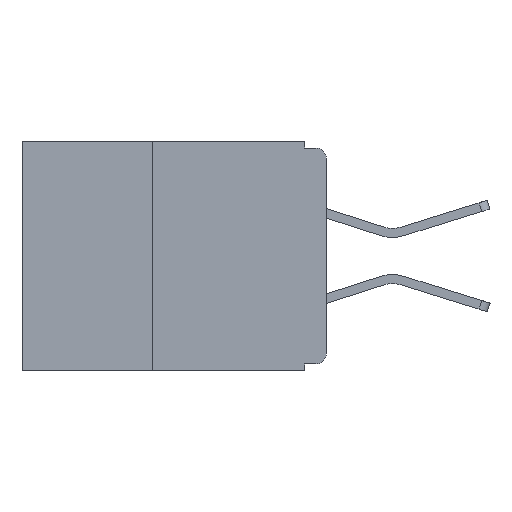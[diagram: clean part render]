
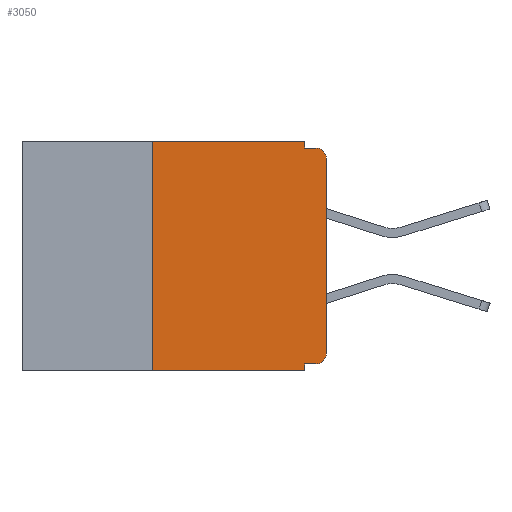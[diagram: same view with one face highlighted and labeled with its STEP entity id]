
A CAD part, left-side view. The second image highlights one B-rep face of the part: STEP entity #3050.
In plain terms, the highlighted planar face has unit normal (-1, 0, 0).
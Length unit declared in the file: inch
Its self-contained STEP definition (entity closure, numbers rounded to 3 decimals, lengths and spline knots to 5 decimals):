
#197 = ORIENTED_EDGE ( 'NONE', *, *, #4888, .F. ) ;
#279 = CARTESIAN_POINT ( 'NONE',  ( 0., 0., -0.01 ) ) ;
#419 = CARTESIAN_POINT ( 'NONE',  ( 0., 0.437, -0.33 ) ) ;
#946 = ORIENTED_EDGE ( 'NONE', *, *, #11681, .T. ) ;
#1035 = VERTEX_POINT ( 'NONE', #1545 ) ;
#1174 = VERTEX_POINT ( 'NONE', #5478 ) ;
#1200 = LINE ( 'NONE', #7722, #11026 ) ;
#1392 = EDGE_CURVE ( 'NONE', #10368, #1035, #6791, .T. ) ;
#1545 = CARTESIAN_POINT ( 'NONE',  ( 0., 0.015, -0.01 ) ) ;
#1683 = CARTESIAN_POINT ( 'NONE',  ( 0., 0., 0. ) ) ;
#1817 = ORIENTED_EDGE ( 'NONE', *, *, #6725, .F. ) ;
#1857 = CARTESIAN_POINT ( 'NONE',  ( 0., 0.437, 0. ) ) ;
#1884 = ORIENTED_EDGE ( 'NONE', *, *, #3184, .F. ) ;
#2213 = DIRECTION ( 'NONE',  ( 0., 0., -1. ) ) ;
#2411 = AXIS2_PLACEMENT_3D ( 'NONE', #9048, #4273, #4188 ) ;
#2417 = CARTESIAN_POINT ( 'NONE',  ( 0., 0., -0.305 ) ) ;
#2438 = CARTESIAN_POINT ( 'NONE',  ( 0., 0.015, -0.32 ) ) ;
#2534 = CARTESIAN_POINT ( 'NONE',  ( 0., 0.031, 0. ) ) ;
#2611 = DIRECTION ( 'NONE',  ( 0., 0., 1. ) ) ;
#2710 = DIRECTION ( 'NONE',  ( 0., 0., -1. ) ) ;
#3050 = ADVANCED_FACE ( 'NONE', ( #4668 ), #9510, .F. ) ;
#3118 = LINE ( 'NONE', #7141, #7321 ) ;
#3184 = EDGE_CURVE ( 'NONE', #4792, #7327, #10621, .T. ) ;
#3186 = AXIS2_PLACEMENT_3D ( 'NONE', #1857, #9550, #2710 ) ;
#3402 = AXIS2_PLACEMENT_3D ( 'NONE', #7175, #7923, #2213 ) ;
#3462 = ORIENTED_EDGE ( 'NONE', *, *, #9249, .T. ) ;
#3850 = CARTESIAN_POINT ( 'NONE',  ( 0., 0., -0.025 ) ) ;
#3907 = LINE ( 'NONE', #419, #4951 ) ;
#4050 = DIRECTION ( 'NONE',  ( 0., 1., 0. ) ) ;
#4117 = CARTESIAN_POINT ( 'NONE',  ( 0., 0.25, -0.33 ) ) ;
#4188 = DIRECTION ( 'NONE',  ( 0., 0., -1. ) ) ;
#4189 = DIRECTION ( 'NONE',  ( 0., -1., 0. ) ) ;
#4273 = DIRECTION ( 'NONE',  ( -1., 0., 0. ) ) ;
#4319 = DIRECTION ( 'NONE',  ( 0., 0., 1. ) ) ;
#4668 = FACE_OUTER_BOUND ( 'NONE', #10624, .T. ) ;
#4792 = VERTEX_POINT ( 'NONE', #7662 ) ;
#4888 = EDGE_CURVE ( 'NONE', #9612, #1174, #6594, .T. ) ;
#4899 = DIRECTION ( 'NONE',  ( 0., 0., -1. ) ) ;
#4951 = VECTOR ( 'NONE', #7119, 39.37008 ) ;
#5375 = VECTOR ( 'NONE', #2611, 39.37008 ) ;
#5478 = CARTESIAN_POINT ( 'NONE',  ( 0., 0.031, -0.32 ) ) ;
#5643 = EDGE_CURVE ( 'NONE', #7419, #12080, #8805, .T. ) ;
#5899 = EDGE_CURVE ( 'NONE', #11147, #4792, #3118, .T. ) ;
#6088 = CARTESIAN_POINT ( 'NONE',  ( 0., 0.031, -0.33 ) ) ;
#6113 = LINE ( 'NONE', #6088, #10429 ) ;
#6269 = CARTESIAN_POINT ( 'NONE',  ( 0., 0.031, -0.33 ) ) ;
#6420 = CIRCLE ( 'NONE', #2411, 0.015 ) ;
#6594 = LINE ( 'NONE', #10680, #10911 ) ;
#6725 = EDGE_CURVE ( 'NONE', #7327, #10368, #1200, .T. ) ;
#6791 = LINE ( 'NONE', #279, #8722 ) ;
#6833 = VERTEX_POINT ( 'NONE', #6269 ) ;
#6882 = DIRECTION ( 'NONE',  ( 0., -1., 0. ) ) ;
#6941 = CIRCLE ( 'NONE', #3402, 0.015 ) ;
#7119 = DIRECTION ( 'NONE',  ( 0., -1., 0. ) ) ;
#7141 = CARTESIAN_POINT ( 'NONE',  ( 0., 0.25, -0.33 ) ) ;
#7151 = ORIENTED_EDGE ( 'NONE', *, *, #1392, .F. ) ;
#7175 = CARTESIAN_POINT ( 'NONE',  ( 0., 0.015, -0.025 ) ) ;
#7182 = DIRECTION ( 'NONE',  ( 0., 0., -1. ) ) ;
#7321 = VECTOR ( 'NONE', #4319, 39.37008 ) ;
#7327 = VERTEX_POINT ( 'NONE', #2534 ) ;
#7419 = VERTEX_POINT ( 'NONE', #2417 ) ;
#7545 = ORIENTED_EDGE ( 'NONE', *, *, #5899, .F. ) ;
#7566 = ORIENTED_EDGE ( 'NONE', *, *, #11706, .F. ) ;
#7662 = CARTESIAN_POINT ( 'NONE',  ( 0., 0.25, 0. ) ) ;
#7676 = ORIENTED_EDGE ( 'NONE', *, *, #5643, .T. ) ;
#7722 = CARTESIAN_POINT ( 'NONE',  ( 0., 0.031, 0. ) ) ;
#7873 = CARTESIAN_POINT ( 'NONE',  ( 0., 0.031, -0.01 ) ) ;
#7923 = DIRECTION ( 'NONE',  ( -1., 0., 0. ) ) ;
#8722 = VECTOR ( 'NONE', #4189, 39.37008 ) ;
#8805 = LINE ( 'NONE', #1683, #5375 ) ;
#9048 = CARTESIAN_POINT ( 'NONE',  ( 0., 0.015, -0.305 ) ) ;
#9249 = EDGE_CURVE ( 'NONE', #12080, #1035, #6941, .T. ) ;
#9510 = PLANE ( 'NONE',  #3186 ) ;
#9550 = DIRECTION ( 'NONE',  ( 1., 0., 0. ) ) ;
#9612 = VERTEX_POINT ( 'NONE', #2438 ) ;
#10368 = VERTEX_POINT ( 'NONE', #7873 ) ;
#10429 = VECTOR ( 'NONE', #7182, 39.37008 ) ;
#10468 = EDGE_CURVE ( 'NONE', #11147, #6833, #3907, .T. ) ;
#10546 = ORIENTED_EDGE ( 'NONE', *, *, #10468, .T. ) ;
#10621 = LINE ( 'NONE', #11627, #11976 ) ;
#10624 = EDGE_LOOP ( 'NONE', ( #7676, #3462, #7151, #1817, #1884, #7545, #10546, #7566, #197, #946 ) ) ;
#10680 = CARTESIAN_POINT ( 'NONE',  ( 0., 0., -0.32 ) ) ;
#10911 = VECTOR ( 'NONE', #4050, 39.37008 ) ;
#11026 = VECTOR ( 'NONE', #4899, 39.37008 ) ;
#11147 = VERTEX_POINT ( 'NONE', #4117 ) ;
#11627 = CARTESIAN_POINT ( 'NONE',  ( 0., 0.437, 0. ) ) ;
#11681 = EDGE_CURVE ( 'NONE', #9612, #7419, #6420, .T. ) ;
#11706 = EDGE_CURVE ( 'NONE', #1174, #6833, #6113, .T. ) ;
#11976 = VECTOR ( 'NONE', #6882, 39.37008 ) ;
#12080 = VERTEX_POINT ( 'NONE', #3850 ) ;
